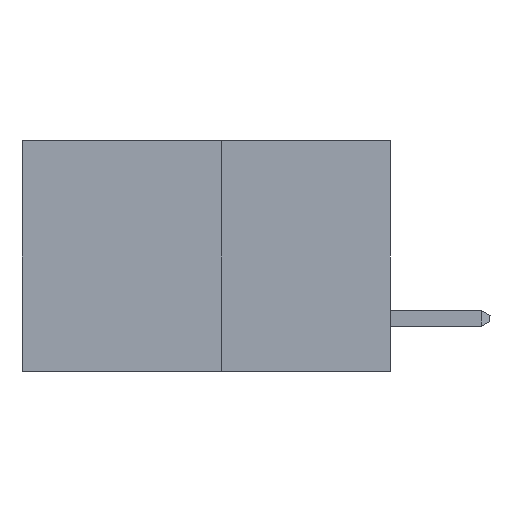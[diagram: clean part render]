
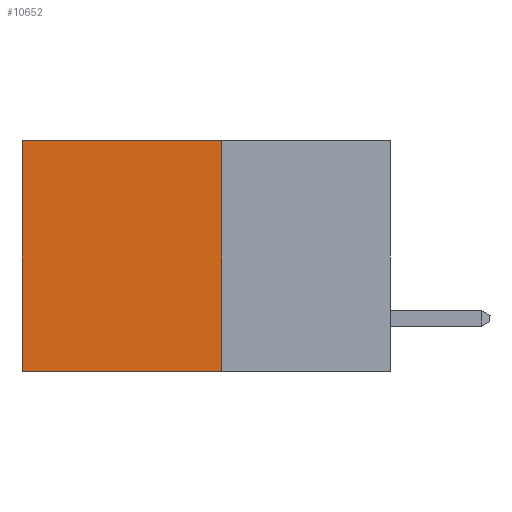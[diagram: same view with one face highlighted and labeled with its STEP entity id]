
A CAD part, left-side view. The second image highlights one B-rep face of the part: STEP entity #10652.
In plain terms, the highlighted planar face has unit normal (-1, 0, 0).
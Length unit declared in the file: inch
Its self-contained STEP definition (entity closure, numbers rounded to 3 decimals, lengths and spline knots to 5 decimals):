
#180 = CARTESIAN_POINT ( 'NONE',  ( 0.277, 0.27, 0. ) ) ;
#443 = DIRECTION ( 'NONE',  ( 0., 0., -1. ) ) ;
#617 = EDGE_LOOP ( 'NONE', ( #1116, #1125, #1157, #1223 ) ) ;
#788 = CARTESIAN_POINT ( 'NONE',  ( 0.277, 0.59, -0.37 ) ) ;
#1116 = ORIENTED_EDGE ( 'NONE', *, *, #5957, .T. ) ;
#1125 = ORIENTED_EDGE ( 'NONE', *, *, #3615, .F. ) ;
#1157 = ORIENTED_EDGE ( 'NONE', *, *, #4385, .F. ) ;
#1223 = ORIENTED_EDGE ( 'NONE', *, *, #5144, .T. ) ;
#2458 = LINE ( 'NONE', #180, #6506 ) ;
#2641 = DIRECTION ( 'NONE',  ( 1., 0., 0. ) ) ;
#3238 = VERTEX_POINT ( 'NONE', #6935 ) ;
#3615 = EDGE_CURVE ( 'NONE', #5021, #3238, #10344, .T. ) ;
#4385 = EDGE_CURVE ( 'NONE', #6978, #5021, #10318, .T. ) ;
#5021 = VERTEX_POINT ( 'NONE', #8205 ) ;
#5144 = EDGE_CURVE ( 'NONE', #6978, #6606, #2458, .T. ) ;
#5201 = CARTESIAN_POINT ( 'NONE',  ( 0.277, 0.27, 0. ) ) ;
#5865 = VECTOR ( 'NONE', #8340, 39.37008 ) ;
#5957 = EDGE_CURVE ( 'NONE', #6606, #3238, #8959, .T. ) ;
#6076 = CARTESIAN_POINT ( 'NONE',  ( 0.277, 0.27, -0.37 ) ) ;
#6234 = CARTESIAN_POINT ( 'NONE',  ( 0.277, 0.27, -0.37 ) ) ;
#6506 = VECTOR ( 'NONE', #7108, 39.37008 ) ;
#6606 = VERTEX_POINT ( 'NONE', #9504 ) ;
#6741 = VECTOR ( 'NONE', #443, 39.37008 ) ;
#6923 = PLANE ( 'NONE',  #9316 ) ;
#6935 = CARTESIAN_POINT ( 'NONE',  ( 0.277, 0.59, -0.37 ) ) ;
#6978 = VERTEX_POINT ( 'NONE', #5201 ) ;
#7108 = DIRECTION ( 'NONE',  ( 0., 1., 0. ) ) ;
#7580 = VECTOR ( 'NONE', #11090, 39.37008 ) ;
#8205 = CARTESIAN_POINT ( 'NONE',  ( 0.277, 0.27, -0.37 ) ) ;
#8340 = DIRECTION ( 'NONE',  ( 0., 1., 0. ) ) ;
#8383 = CARTESIAN_POINT ( 'NONE',  ( 0.277, 0.27, -0.37 ) ) ;
#8582 = DIRECTION ( 'NONE',  ( 0., 0., -1. ) ) ;
#8959 = LINE ( 'NONE', #788, #6741 ) ;
#9316 = AXIS2_PLACEMENT_3D ( 'NONE', #6076, #2641, #8582 ) ;
#9504 = CARTESIAN_POINT ( 'NONE',  ( 0.277, 0.59, 0. ) ) ;
#10318 = LINE ( 'NONE', #6234, #7580 ) ;
#10344 = LINE ( 'NONE', #8383, #5865 ) ;
#10587 = FACE_OUTER_BOUND ( 'NONE', #617, .T. ) ;
#10652 = ADVANCED_FACE ( 'NONE', ( #10587 ), #6923, .F. ) ;
#11090 = DIRECTION ( 'NONE',  ( 0., 0., -1. ) ) ;
